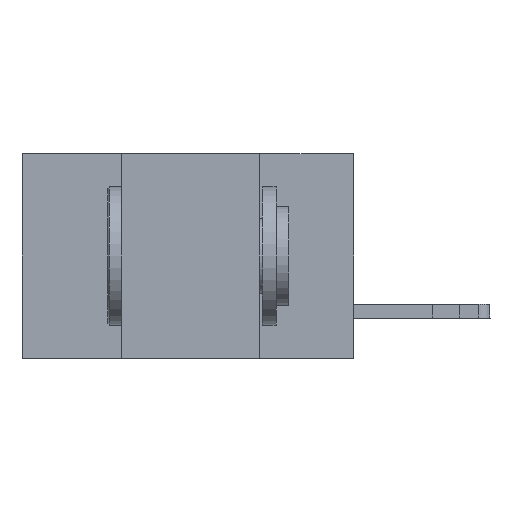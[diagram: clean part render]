
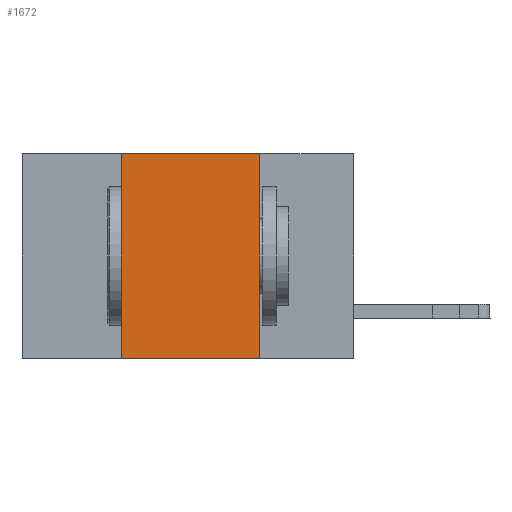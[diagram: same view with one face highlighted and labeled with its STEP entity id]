
A CAD part, left-side view. The second image highlights one B-rep face of the part: STEP entity #1672.
In plain terms, the highlighted planar face has unit normal (-1, 0, 0).
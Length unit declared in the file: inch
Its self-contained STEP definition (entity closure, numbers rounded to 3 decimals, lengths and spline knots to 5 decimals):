
#1672 = ADVANCED_FACE ( 'NONE', ( #12193 ), #16000, .F. ) ;
#2053 = VERTEX_POINT ( 'NONE', #8980 ) ;
#2288 = CARTESIAN_POINT ( 'NONE',  ( 0., 0.6, 0. ) ) ;
#2797 = CARTESIAN_POINT ( 'NONE',  ( 0., 0.6, -0.37 ) ) ;
#2909 = ORIENTED_EDGE ( 'NONE', *, *, #18710, .F. ) ;
#3682 = LINE ( 'NONE', #2288, #15776 ) ;
#3986 = VECTOR ( 'NONE', #15220, 39.37008 ) ;
#4266 = DIRECTION ( 'NONE',  ( 0., -1., 0. ) ) ;
#5007 = EDGE_LOOP ( 'NONE', ( #6077, #2909, #7319, #11858 ) ) ;
#5018 = CARTESIAN_POINT ( 'NONE',  ( 0., 0.42, 0. ) ) ;
#6077 = ORIENTED_EDGE ( 'NONE', *, *, #17959, .F. ) ;
#6746 = VECTOR ( 'NONE', #12289, 39.37008 ) ;
#7319 = ORIENTED_EDGE ( 'NONE', *, *, #13280, .F. ) ;
#8059 = VECTOR ( 'NONE', #4266, 39.37008 ) ;
#8534 = LINE ( 'NONE', #2797, #8059 ) ;
#8980 = CARTESIAN_POINT ( 'NONE',  ( 0., 0.42, -0.37 ) ) ;
#9767 = EDGE_CURVE ( 'NONE', #2053, #14169, #8534, .T. ) ;
#11858 = ORIENTED_EDGE ( 'NONE', *, *, #9767, .T. ) ;
#12193 = FACE_OUTER_BOUND ( 'NONE', #5007, .T. ) ;
#12289 = DIRECTION ( 'NONE',  ( 0., 0., -1. ) ) ;
#12579 = DIRECTION ( 'NONE',  ( 0., -1., 0. ) ) ;
#13222 = VERTEX_POINT ( 'NONE', #16449 ) ;
#13280 = EDGE_CURVE ( 'NONE', #2053, #18238, #15187, .T. ) ;
#14169 = VERTEX_POINT ( 'NONE', #15801 ) ;
#14504 = LINE ( 'NONE', #17857, #6746 ) ;
#15187 = LINE ( 'NONE', #5018, #3986 ) ;
#15220 = DIRECTION ( 'NONE',  ( 0., 0., 1. ) ) ;
#15776 = VECTOR ( 'NONE', #12579, 39.37008 ) ;
#15801 = CARTESIAN_POINT ( 'NONE',  ( 0., 0.17, -0.37 ) ) ;
#16000 = PLANE ( 'NONE',  #16731 ) ;
#16177 = CARTESIAN_POINT ( 'NONE',  ( 0., 0.6, 0. ) ) ;
#16262 = DIRECTION ( 'NONE',  ( 0., 0., -1. ) ) ;
#16279 = DIRECTION ( 'NONE',  ( 1., 0., 0. ) ) ;
#16449 = CARTESIAN_POINT ( 'NONE',  ( 0., 0.17, 0. ) ) ;
#16731 = AXIS2_PLACEMENT_3D ( 'NONE', #16177, #16279, #16262 ) ;
#17129 = CARTESIAN_POINT ( 'NONE',  ( 0., 0.42, 0. ) ) ;
#17857 = CARTESIAN_POINT ( 'NONE',  ( 0., 0.17, 0. ) ) ;
#17959 = EDGE_CURVE ( 'NONE', #13222, #14169, #14504, .T. ) ;
#18238 = VERTEX_POINT ( 'NONE', #17129 ) ;
#18710 = EDGE_CURVE ( 'NONE', #18238, #13222, #3682, .T. ) ;
